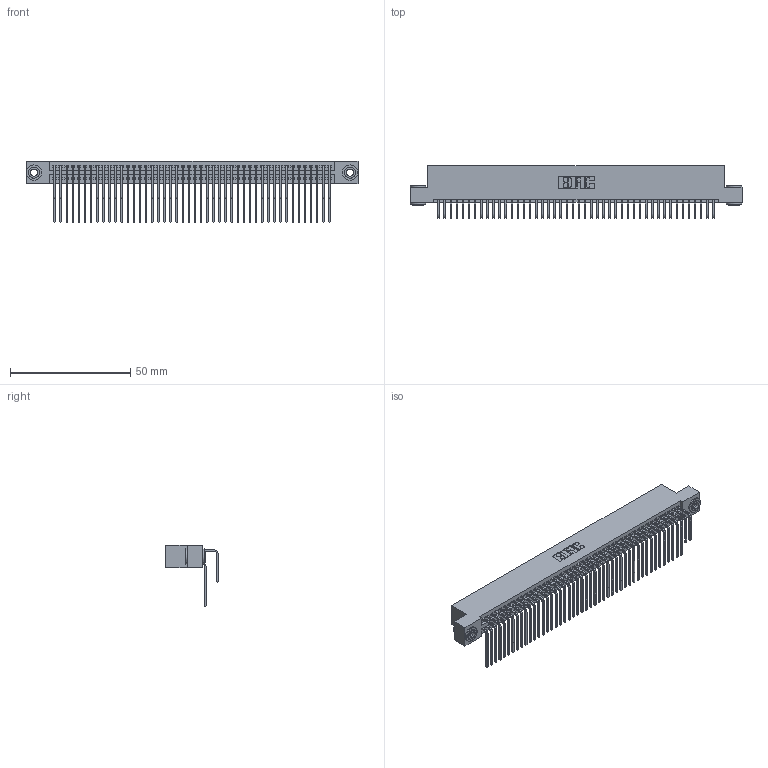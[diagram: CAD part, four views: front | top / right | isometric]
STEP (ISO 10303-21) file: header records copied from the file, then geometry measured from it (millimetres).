
FILE_DESCRIPTION (( 'STEP AP203' ), '1' );
FILE_NAME ('395-092-558-203.STEP', '2019-10-25T20:27:19', ( '' ), ( '' ), 'SwSTEP 2.0', 'SolidWorks 2016', '' );
FILE_SCHEMA (( 'CONFIG_CONTROL_DESIGN' ));
Length unit declared in the file: inch
Products named in the file (5): 345-292-001_558 559 Tail - 1; 345-292-001_558 Tail - 2; 345-250-002_345-250-002-102; 395-092-558-203; 345 Part_Flush Mounting Lugs - 0.156 Dia-TH
Assembly tree (95 placements, depth 2):
  395-092-558-203
    345 Part_Flush Mounting Lugs - 0.156 Dia-TH
    345-292-001_558 559 Tail - 1  x46
    345-292-001_558 Tail - 2  x46
    345-250-002_345-250-002-102  x2
Bounding box: 138.05 x 21.83 x 25.53 mm (x, y, z)
Volume: 13997.5 mm3; surface area: 23468.6 mm2
Topology: 95 solids, 95 shells, 4948 faces, 14677 edges, 9658 vertices
Faces by surface type: plane 3310, cylinder 1630, cone 8
Entity records: 37856 total; most frequent: CARTESIAN_POINT 6362, ORIENTED_EDGE 6238, DIRECTION 5609, EDGE_CURVE 3119, LINE 2739, VECTOR 2739, VERTEX_POINT 2074, AXIS2_PLACEMENT_3D 1435
